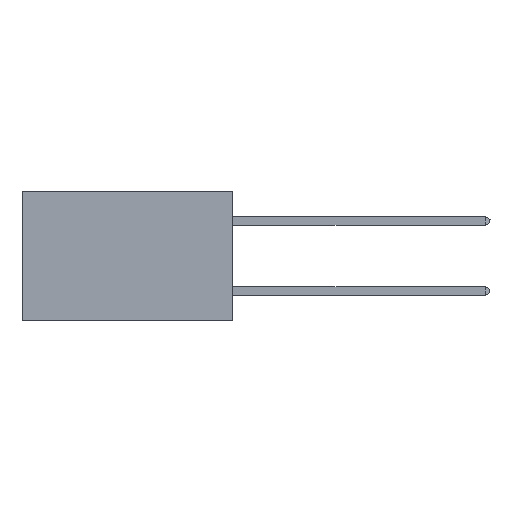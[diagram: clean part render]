
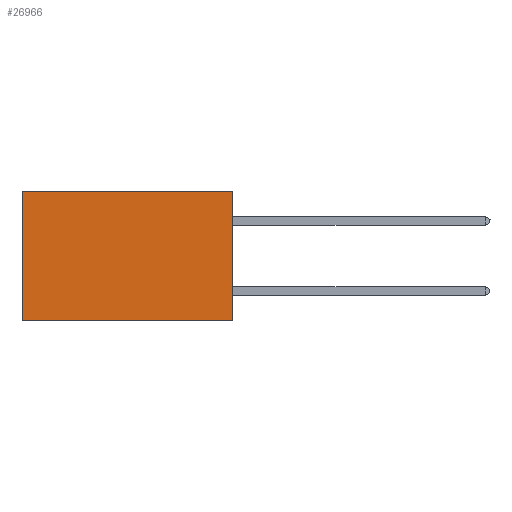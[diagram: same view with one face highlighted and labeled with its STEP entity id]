
A CAD part, left-side view. The second image highlights one B-rep face of the part: STEP entity #26966.
In plain terms, the highlighted planar face has unit normal (-1, 0, 0).
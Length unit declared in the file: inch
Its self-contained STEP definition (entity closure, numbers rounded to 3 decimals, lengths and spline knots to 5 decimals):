
#603 = CARTESIAN_POINT ( 'NONE',  ( 0.2875, 0.6, 0. ) ) ;
#1212 = EDGE_CURVE ( 'NONE', #17883, #25038, #2215, .T. ) ;
#1405 = CARTESIAN_POINT ( 'NONE',  ( 0.2875, 0.6, 0. ) ) ;
#2215 = LINE ( 'NONE', #22608, #4317 ) ;
#2347 = DIRECTION ( 'NONE',  ( 1., 0., 0. ) ) ;
#2528 = DIRECTION ( 'NONE',  ( 0., 0., -1. ) ) ;
#2964 = AXIS2_PLACEMENT_3D ( 'NONE', #20071, #2347, #8993 ) ;
#4317 = VECTOR ( 'NONE', #7242, 39.37008 ) ;
#4519 = CARTESIAN_POINT ( 'NONE',  ( 0.2875, 0., -0.37 ) ) ;
#5728 = ORIENTED_EDGE ( 'NONE', *, *, #15480, .F. ) ;
#6970 = EDGE_LOOP ( 'NONE', ( #22355, #5728, #19921, #18155 ) ) ;
#7242 = DIRECTION ( 'NONE',  ( 0., 1., 0. ) ) ;
#7765 = FACE_OUTER_BOUND ( 'NONE', #6970, .T. ) ;
#8633 = CARTESIAN_POINT ( 'NONE',  ( 0.2875, 0.6, -0.37 ) ) ;
#8993 = DIRECTION ( 'NONE',  ( 0., 0., -1. ) ) ;
#9080 = LINE ( 'NONE', #24424, #23574 ) ;
#9625 = VECTOR ( 'NONE', #2528, 39.37008 ) ;
#11067 = VERTEX_POINT ( 'NONE', #8633 ) ;
#11143 = CARTESIAN_POINT ( 'NONE',  ( 0.2875, 0., -0.37 ) ) ;
#11266 = DIRECTION ( 'NONE',  ( 0., 1., 0. ) ) ;
#13628 = PLANE ( 'NONE',  #2964 ) ;
#13924 = LINE ( 'NONE', #4519, #19467 ) ;
#15480 = EDGE_CURVE ( 'NONE', #21111, #11067, #13924, .T. ) ;
#16045 = EDGE_CURVE ( 'NONE', #17883, #21111, #9080, .T. ) ;
#17883 = VERTEX_POINT ( 'NONE', #20743 ) ;
#18155 = ORIENTED_EDGE ( 'NONE', *, *, #1212, .T. ) ;
#19467 = VECTOR ( 'NONE', #11266, 39.37008 ) ;
#19891 = DIRECTION ( 'NONE',  ( 0., 0., -1. ) ) ;
#19916 = EDGE_CURVE ( 'NONE', #25038, #11067, #24119, .T. ) ;
#19921 = ORIENTED_EDGE ( 'NONE', *, *, #16045, .F. ) ;
#20071 = CARTESIAN_POINT ( 'NONE',  ( 0.2875, 0., 0. ) ) ;
#20743 = CARTESIAN_POINT ( 'NONE',  ( 0.2875, 0., 0. ) ) ;
#21111 = VERTEX_POINT ( 'NONE', #11143 ) ;
#22355 = ORIENTED_EDGE ( 'NONE', *, *, #19916, .T. ) ;
#22608 = CARTESIAN_POINT ( 'NONE',  ( 0.2875, 0., 0. ) ) ;
#23574 = VECTOR ( 'NONE', #19891, 39.37008 ) ;
#24119 = LINE ( 'NONE', #603, #9625 ) ;
#24424 = CARTESIAN_POINT ( 'NONE',  ( 0.2875, 0., 0. ) ) ;
#25038 = VERTEX_POINT ( 'NONE', #1405 ) ;
#26966 = ADVANCED_FACE ( 'NONE', ( #7765 ), #13628, .F. ) ;
